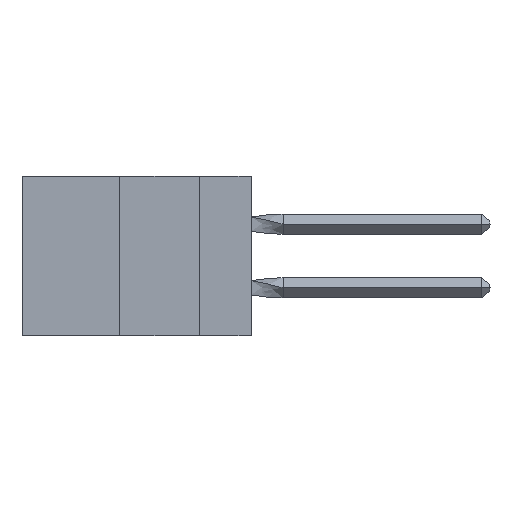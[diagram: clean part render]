
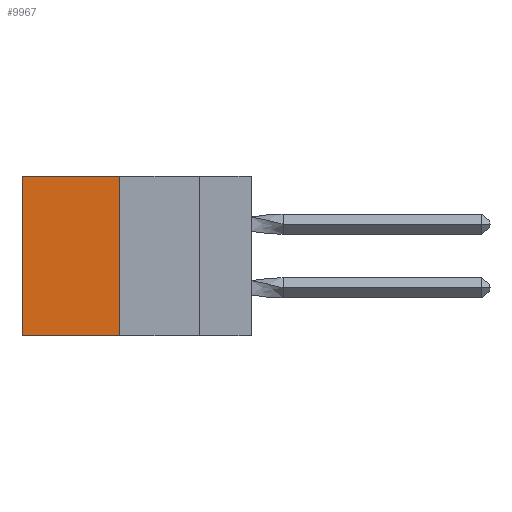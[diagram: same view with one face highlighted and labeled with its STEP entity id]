
A CAD part, left-side view. The second image highlights one B-rep face of the part: STEP entity #9967.
In plain terms, the highlighted planar face has unit normal (-1, 0, 0).
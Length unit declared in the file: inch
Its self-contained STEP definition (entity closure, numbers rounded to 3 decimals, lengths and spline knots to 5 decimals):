
#184 = ORIENTED_EDGE ( 'NONE', *, *, #2347, .F. ) ;
#261 = VERTEX_POINT ( 'NONE', #1024 ) ;
#1024 = CARTESIAN_POINT ( 'NONE',  ( 0.305, 0.413, -0.5 ) ) ;
#1255 = CARTESIAN_POINT ( 'NONE',  ( 0.305, 0.72, 0. ) ) ;
#1402 = CARTESIAN_POINT ( 'NONE',  ( 0.305, 0.72, -0.5 ) ) ;
#1557 = LINE ( 'NONE', #2132, #2615 ) ;
#2132 = CARTESIAN_POINT ( 'NONE',  ( 0.305, 0.413, -0.5 ) ) ;
#2347 = EDGE_CURVE ( 'NONE', #13441, #261, #3598, .T. ) ;
#2576 = ORIENTED_EDGE ( 'NONE', *, *, #13327, .T. ) ;
#2615 = VECTOR ( 'NONE', #5035, 39.37008 ) ;
#3003 = PLANE ( 'NONE',  #9461 ) ;
#3598 = LINE ( 'NONE', #10169, #17619 ) ;
#5035 = DIRECTION ( 'NONE',  ( 0., 1., 0. ) ) ;
#5137 = EDGE_LOOP ( 'NONE', ( #2576, #11506, #184, #11446 ) ) ;
#5386 = DIRECTION ( 'NONE',  ( 0., 0., -1. ) ) ;
#6767 = LINE ( 'NONE', #7575, #11023 ) ;
#7575 = CARTESIAN_POINT ( 'NONE',  ( 0.305, 0.413, 0. ) ) ;
#9461 = AXIS2_PLACEMENT_3D ( 'NONE', #13236, #12518, #17073 ) ;
#9606 = FACE_OUTER_BOUND ( 'NONE', #5137, .T. ) ;
#9649 = VERTEX_POINT ( 'NONE', #1255 ) ;
#9967 = ADVANCED_FACE ( 'NONE', ( #9606 ), #3003, .F. ) ;
#10169 = CARTESIAN_POINT ( 'NONE',  ( 0.305, 0.413, -0.5 ) ) ;
#10805 = CARTESIAN_POINT ( 'NONE',  ( 0.305, 0.72, -0.5 ) ) ;
#11023 = VECTOR ( 'NONE', #12949, 39.37008 ) ;
#11446 = ORIENTED_EDGE ( 'NONE', *, *, #14482, .T. ) ;
#11506 = ORIENTED_EDGE ( 'NONE', *, *, #13058, .F. ) ;
#12518 = DIRECTION ( 'NONE',  ( 1., 0., 0. ) ) ;
#12949 = DIRECTION ( 'NONE',  ( 0., 1., 0. ) ) ;
#13058 = EDGE_CURVE ( 'NONE', #261, #16204, #1557, .T. ) ;
#13236 = CARTESIAN_POINT ( 'NONE',  ( 0.305, 0.413, -0.5 ) ) ;
#13327 = EDGE_CURVE ( 'NONE', #9649, #16204, #14776, .T. ) ;
#13441 = VERTEX_POINT ( 'NONE', #15147 ) ;
#14482 = EDGE_CURVE ( 'NONE', #13441, #9649, #6767, .T. ) ;
#14776 = LINE ( 'NONE', #1402, #16652 ) ;
#15147 = CARTESIAN_POINT ( 'NONE',  ( 0.305, 0.413, 0. ) ) ;
#16003 = DIRECTION ( 'NONE',  ( 0., 0., -1. ) ) ;
#16204 = VERTEX_POINT ( 'NONE', #10805 ) ;
#16652 = VECTOR ( 'NONE', #5386, 39.37008 ) ;
#17073 = DIRECTION ( 'NONE',  ( 0., 0., -1. ) ) ;
#17619 = VECTOR ( 'NONE', #16003, 39.37008 ) ;
